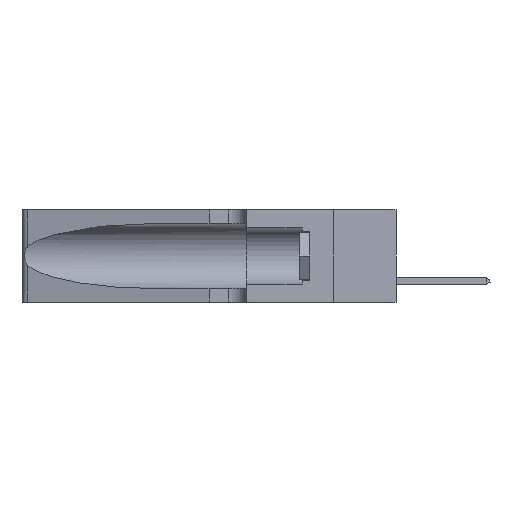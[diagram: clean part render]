
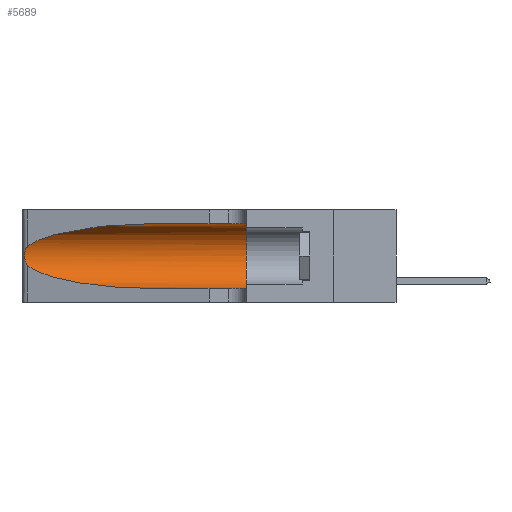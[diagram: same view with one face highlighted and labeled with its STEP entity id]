
A CAD part, left-side view. The second image highlights one B-rep face of the part: STEP entity #5689.
In plain terms, the highlighted cylindrical face has radius 3.308 mm (diameter 6.617 mm), a partial arc.
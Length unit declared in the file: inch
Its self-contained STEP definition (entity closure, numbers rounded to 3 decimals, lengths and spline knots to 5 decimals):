
#545 = CARTESIAN_POINT ( 'NONE',  ( 0.1305, 0.35, 0.185 ) ) ;
#1037 = VERTEX_POINT ( 'NONE', #16807 ) ;
#1783 = EDGE_CURVE ( 'NONE', #2403, #1037, #10757, .T. ) ;
#2174 = EDGE_LOOP ( 'NONE', ( #27652, #30039, #16121, #28523, #3126, #5303 ) ) ;
#2218 = CARTESIAN_POINT ( 'NONE',  ( 0.25487, 1.22718, 0.22369 ) ) ;
#2320 = CARTESIAN_POINT ( 'NONE',  ( 0.25555, 1.22994, 0.2215 ) ) ;
#2403 = VERTEX_POINT ( 'NONE', #4692 ) ;
#2603 = VERTEX_POINT ( 'NONE', #25829 ) ;
#2635 = EDGE_CURVE ( 'NONE', #9531, #2603, #18887, .T. ) ;
#3126 = ORIENTED_EDGE ( 'NONE', *, *, #2635, .F. ) ;
#3333 = CARTESIAN_POINT ( 'NONE',  ( 0.2373, 1.15595, 0.08982 ) ) ;
#3736 = AXIS2_PLACEMENT_3D ( 'NONE', #545, #28789, #14924 ) ;
#3800 = EDGE_CURVE ( 'NONE', #1037, #2603, #20985, .T. ) ;
#4443 = CARTESIAN_POINT ( 'NONE',  ( 0.26017, 1.23833, 0.17102 ) ) ;
#4692 = CARTESIAN_POINT ( 'NONE',  ( 0.25487, 1.22718, 0.14631 ) ) ;
#4697 = CARTESIAN_POINT ( 'NONE',  ( 0.2373, 1.15595, 0.28018 ) ) ;
#4804 = CARTESIAN_POINT ( 'NONE',  ( 0.1305, 0.35, 0.31525 ) ) ;
#5303 = ORIENTED_EDGE ( 'NONE', *, *, #27065, .F. ) ;
#5689 = ADVANCED_FACE ( 'NONE', ( #19805 ), #10716, .F. ) ;
#6783 = CARTESIAN_POINT ( 'NONE',  ( 0.18966, 0.96281, 0.05475 ) ) ;
#6900 = CARTESIAN_POINT ( 'NONE',  ( 0.26075, 1.23896, 0.178 ) ) ;
#7152 = CARTESIAN_POINT ( 'NONE',  ( 0.1305, 0.72297, 0.31525 ) ) ;
#7247 = CARTESIAN_POINT ( 'NONE',  ( 0.18966, 0.96281, 0.31525 ) ) ;
#7914 = VERTEX_POINT ( 'NONE', #21770 ) ;
#8277 = CARTESIAN_POINT ( 'NONE',  ( 0.1305, 1.61858, 0.31525 ) ) ;
#8928 = CARTESIAN_POINT ( 'NONE',  ( 0.25639, 1.23184, 0.21858 ) ) ;
#9531 = VERTEX_POINT ( 'NONE', #4804 ) ;
#10246 = AXIS2_PLACEMENT_3D ( 'NONE', #12607, #22109, #12902 ) ;
#10716 = CYLINDRICAL_SURFACE ( 'NONE', #10246, 0.13025 ) ;
#10757 =( BOUNDED_CURVE ( )  B_SPLINE_CURVE ( 3, ( #17225, #3333, #6783, #25167 ),
 .UNSPECIFIED., .F., .F. ) 
 B_SPLINE_CURVE_WITH_KNOTS ( ( 4, 4 ),
 ( 3.44316, 4.71239 ),
 .UNSPECIFIED. ) 
 CURVE ( )  GEOMETRIC_REPRESENTATION_ITEM ( )  RATIONAL_B_SPLINE_CURVE ( ( 1., 0.87, 0.87, 1. ) ) 
 REPRESENTATION_ITEM ( '' )  );
#11392 = CARTESIAN_POINT ( 'NONE',  ( 0.26018, 1.23835, 0.19895 ) ) ;
#12607 = CARTESIAN_POINT ( 'NONE',  ( 0.1305, 1.61858, 0.185 ) ) ;
#12902 = DIRECTION ( 'NONE',  ( 0., 0., -1. ) ) ;
#13759 = CARTESIAN_POINT ( 'NONE',  ( 0.26075, 1.23896, 0.19203 ) ) ;
#14198 = EDGE_CURVE ( 'NONE', #7914, #2403, #18037, .T. ) ;
#14535 = CARTESIAN_POINT ( 'NONE',  ( 0.1305, 1.61858, 0.05475 ) ) ;
#14823 = VERTEX_POINT ( 'NONE', #20661 ) ;
#14924 = DIRECTION ( 'NONE',  ( 0., 0., 1. ) ) ;
#16121 = ORIENTED_EDGE ( 'NONE', *, *, #1783, .T. ) ;
#16171 =( BOUNDED_CURVE ( )  B_SPLINE_CURVE ( 3, ( #7152, #7247, #4697, #23367 ),
 .UNSPECIFIED., .F., .F. ) 
 B_SPLINE_CURVE_WITH_KNOTS ( ( 4, 4 ),
 ( 1.5708, 2.84003 ),
 .UNSPECIFIED. ) 
 CURVE ( )  GEOMETRIC_REPRESENTATION_ITEM ( )  RATIONAL_B_SPLINE_CURVE ( ( 1., 0.87, 0.87, 1. ) ) 
 REPRESENTATION_ITEM ( '' )  );
#16807 = CARTESIAN_POINT ( 'NONE',  ( 0.1305, 0.72297, 0.05475 ) ) ;
#17225 = CARTESIAN_POINT ( 'NONE',  ( 0.25487, 1.22718, 0.14631 ) ) ;
#18037 = B_SPLINE_CURVE_WITH_KNOTS ( 'NONE', 3,
 ( #2218, #2320, #8928, #18614, #25460, #11392, #13759, #6900, #4443, #29960, #30059, #20921, #18518, #20741 ),
 .UNSPECIFIED., .F., .F.,
 ( 4, 2, 2, 2, 2, 2, 4 ),
 ( 0., 0.00027, 0.00053, 0.00107, 0.0016, 0.00187, 0.00214 ),
 .UNSPECIFIED. ) ;
#18518 = CARTESIAN_POINT ( 'NONE',  ( 0.25555, 1.22993, 0.14849 ) ) ;
#18614 = CARTESIAN_POINT ( 'NONE',  ( 0.25787, 1.23484, 0.2124 ) ) ;
#18667 = VECTOR ( 'NONE', #20077, 39.37008 ) ;
#18887 = CIRCLE ( 'NONE', #3736, 0.13025 ) ;
#19390 = DIRECTION ( 'NONE',  ( 0., -1., 0. ) ) ;
#19805 = FACE_OUTER_BOUND ( 'NONE', #2174, .T. ) ;
#20077 = DIRECTION ( 'NONE',  ( 0., -1., 0. ) ) ;
#20455 = EDGE_CURVE ( 'NONE', #14823, #7914, #16171, .T. ) ;
#20661 = CARTESIAN_POINT ( 'NONE',  ( 0.1305, 0.72297, 0.31525 ) ) ;
#20741 = CARTESIAN_POINT ( 'NONE',  ( 0.25487, 1.22718, 0.14631 ) ) ;
#20921 = CARTESIAN_POINT ( 'NONE',  ( 0.25639, 1.23186, 0.15144 ) ) ;
#20985 = LINE ( 'NONE', #14535, #28634 ) ;
#21770 = CARTESIAN_POINT ( 'NONE',  ( 0.25487, 1.22718, 0.22369 ) ) ;
#22109 = DIRECTION ( 'NONE',  ( 0., -1., 0. ) ) ;
#23367 = CARTESIAN_POINT ( 'NONE',  ( 0.25487, 1.22718, 0.22369 ) ) ;
#24790 = LINE ( 'NONE', #8277, #18667 ) ;
#25167 = CARTESIAN_POINT ( 'NONE',  ( 0.1305, 0.72297, 0.05475 ) ) ;
#25460 = CARTESIAN_POINT ( 'NONE',  ( 0.25854, 1.2359, 0.20912 ) ) ;
#25829 = CARTESIAN_POINT ( 'NONE',  ( 0.1305, 0.35, 0.05475 ) ) ;
#27065 = EDGE_CURVE ( 'NONE', #14823, #9531, #24790, .T. ) ;
#27652 = ORIENTED_EDGE ( 'NONE', *, *, #20455, .T. ) ;
#28523 = ORIENTED_EDGE ( 'NONE', *, *, #3800, .T. ) ;
#28634 = VECTOR ( 'NONE', #19390, 39.37008 ) ;
#28789 = DIRECTION ( 'NONE',  ( 0., 1., 0. ) ) ;
#29960 = CARTESIAN_POINT ( 'NONE',  ( 0.25856, 1.23593, 0.16098 ) ) ;
#30039 = ORIENTED_EDGE ( 'NONE', *, *, #14198, .T. ) ;
#30059 = CARTESIAN_POINT ( 'NONE',  ( 0.25789, 1.23486, 0.15765 ) ) ;
